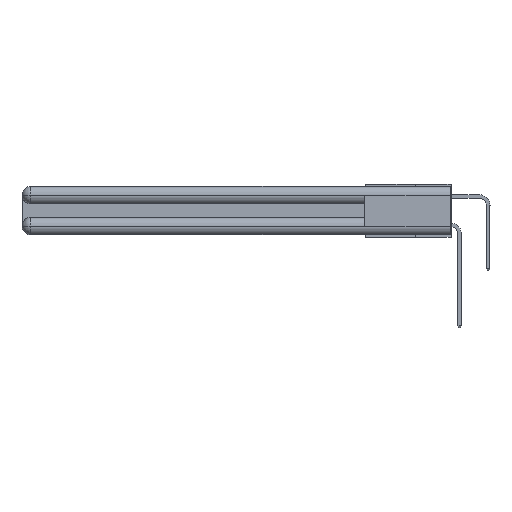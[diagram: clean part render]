
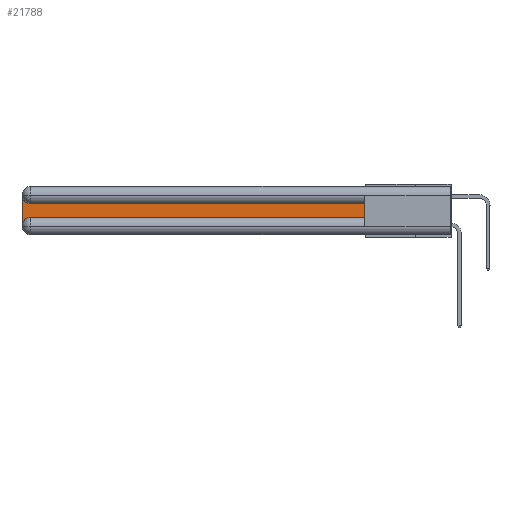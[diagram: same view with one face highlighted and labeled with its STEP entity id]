
A CAD part, left-side view. The second image highlights one B-rep face of the part: STEP entity #21788.
In plain terms, the highlighted planar face has unit normal (-1, 0, 0).
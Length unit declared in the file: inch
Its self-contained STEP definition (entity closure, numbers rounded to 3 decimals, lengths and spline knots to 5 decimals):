
#72 = VERTEX_POINT ( 'NONE', #27974 ) ;
#568 = EDGE_CURVE ( 'NONE', #8370, #72, #24254, .T. ) ;
#1173 = ORIENTED_EDGE ( 'NONE', *, *, #568, .T. ) ;
#2162 = ORIENTED_EDGE ( 'NONE', *, *, #17916, .T. ) ;
#2798 = FACE_OUTER_BOUND ( 'NONE', #7677, .T. ) ;
#4078 = ORIENTED_EDGE ( 'NONE', *, *, #17061, .T. ) ;
#5101 = LINE ( 'NONE', #21076, #18121 ) ;
#5826 = AXIS2_PLACEMENT_3D ( 'NONE', #29063, #20331, #26693 ) ;
#6459 = VERTEX_POINT ( 'NONE', #9442 ) ;
#6850 = CIRCLE ( 'NONE', #27523, 0.06 ) ;
#7255 = ORIENTED_EDGE ( 'NONE', *, *, #26059, .T. ) ;
#7588 = DIRECTION ( 'NONE',  ( 0., 0., -1. ) ) ;
#7677 = EDGE_LOOP ( 'NONE', ( #7255, #26780, #2162, #12295, #4078, #1173 ) ) ;
#8370 = VERTEX_POINT ( 'NONE', #27240 ) ;
#8750 = VECTOR ( 'NONE', #13868, 39.37008 ) ;
#9442 = CARTESIAN_POINT ( 'NONE',  ( 0.075, 3., -0.2775 ) ) ;
#9519 = EDGE_CURVE ( 'NONE', #20001, #23305, #26621, .T. ) ;
#9839 = DIRECTION ( 'NONE',  ( 0., -1., 0. ) ) ;
#10143 = CARTESIAN_POINT ( 'NONE',  ( 0.075, 2.94, -0.1225 ) ) ;
#10434 = DIRECTION ( 'NONE',  ( 0., 0., -1. ) ) ;
#10715 = CARTESIAN_POINT ( 'NONE',  ( 0.075, 2.94, -0.2775 ) ) ;
#12295 = ORIENTED_EDGE ( 'NONE', *, *, #15288, .T. ) ;
#12861 = DIRECTION ( 'NONE',  ( 1., 0., 0. ) ) ;
#13400 = PLANE ( 'NONE',  #5826 ) ;
#13527 = AXIS2_PLACEMENT_3D ( 'NONE', #23969, #19410, #10434 ) ;
#13868 = DIRECTION ( 'NONE',  ( 0., 1., 0. ) ) ;
#14948 = CARTESIAN_POINT ( 'NONE',  ( 0.075, 2.94, -0.2175 ) ) ;
#15046 = VECTOR ( 'NONE', #25639, 39.37008 ) ;
#15110 = LINE ( 'NONE', #22789, #8750 ) ;
#15288 = EDGE_CURVE ( 'NONE', #6459, #24674, #6850, .T. ) ;
#16350 = CARTESIAN_POINT ( 'NONE',  ( 0.075, 3., -0.0625 ) ) ;
#17061 = EDGE_CURVE ( 'NONE', #24674, #8370, #18017, .T. ) ;
#17916 = EDGE_CURVE ( 'NONE', #23305, #6459, #5101, .T. ) ;
#18017 = LINE ( 'NONE', #21085, #26903 ) ;
#18121 = VECTOR ( 'NONE', #7588, 39.37008 ) ;
#19410 = DIRECTION ( 'NONE',  ( 1., 0., 0. ) ) ;
#20001 = VERTEX_POINT ( 'NONE', #10143 ) ;
#20331 = DIRECTION ( 'NONE',  ( 1., 0., 0. ) ) ;
#21076 = CARTESIAN_POINT ( 'NONE',  ( 0.075, 3., -0.2175 ) ) ;
#21085 = CARTESIAN_POINT ( 'NONE',  ( 0.075, 0.6, -0.2175 ) ) ;
#21174 = CARTESIAN_POINT ( 'NONE',  ( 0.075, 0.6, -0.2175 ) ) ;
#21788 = ADVANCED_FACE ( 'NONE', ( #2798 ), #13400, .F. ) ;
#22789 = CARTESIAN_POINT ( 'NONE',  ( 0.075, 0.6, -0.1225 ) ) ;
#23305 = VERTEX_POINT ( 'NONE', #16350 ) ;
#23969 = CARTESIAN_POINT ( 'NONE',  ( 0.075, 2.94, -0.0625 ) ) ;
#24252 = DIRECTION ( 'NONE',  ( 0., 0., -1. ) ) ;
#24254 = LINE ( 'NONE', #21174, #15046 ) ;
#24674 = VERTEX_POINT ( 'NONE', #14948 ) ;
#25639 = DIRECTION ( 'NONE',  ( 0., 0., 1. ) ) ;
#26059 = EDGE_CURVE ( 'NONE', #72, #20001, #15110, .T. ) ;
#26621 = CIRCLE ( 'NONE', #13527, 0.06 ) ;
#26693 = DIRECTION ( 'NONE',  ( 0., 0., -1. ) ) ;
#26780 = ORIENTED_EDGE ( 'NONE', *, *, #9519, .T. ) ;
#26903 = VECTOR ( 'NONE', #9839, 39.37008 ) ;
#27240 = CARTESIAN_POINT ( 'NONE',  ( 0.075, 0.6, -0.2175 ) ) ;
#27523 = AXIS2_PLACEMENT_3D ( 'NONE', #10715, #12861, #24252 ) ;
#27974 = CARTESIAN_POINT ( 'NONE',  ( 0.075, 0.6, -0.1225 ) ) ;
#29063 = CARTESIAN_POINT ( 'NONE',  ( 0.075, 3., -0.1225 ) ) ;
